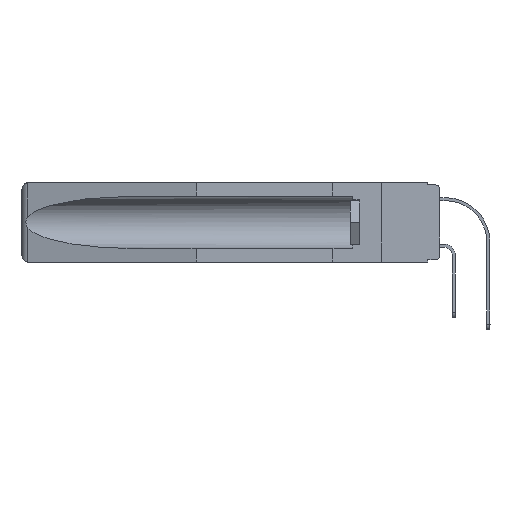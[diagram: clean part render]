
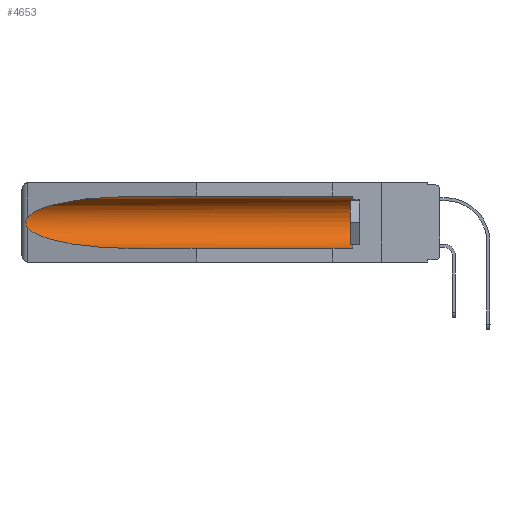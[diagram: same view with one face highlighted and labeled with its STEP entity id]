
A CAD part, left-side view. The second image highlights one B-rep face of the part: STEP entity #4653.
In plain terms, the highlighted cylindrical face has radius 2.857 mm (diameter 5.715 mm), a partial arc.
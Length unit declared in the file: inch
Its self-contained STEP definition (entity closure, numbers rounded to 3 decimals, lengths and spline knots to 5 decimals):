
#161 = ORIENTED_EDGE ( 'NONE', *, *, #1066, .T. ) ;
#438 = CARTESIAN_POINT ( 'NONE',  ( 0.26654, 1.53092, -0.15636 ) ) ;
#1066 = EDGE_CURVE ( 'NONE', #9084, #10188, #7623, .T. ) ;
#1210 = DIRECTION ( 'NONE',  ( 0., -1., 0. ) ) ;
#2127 = VECTOR ( 'NONE', #6569, 39.37008 ) ;
#2269 = ORIENTED_EDGE ( 'NONE', *, *, #20257, .T. ) ;
#2356 = CARTESIAN_POINT ( 'NONE',  ( 0.26537, 1.52718, -0.19328 ) ) ;
#2410 = EDGE_LOOP ( 'NONE', ( #161, #15070, #22019, #6630, #9213, #2269 ) ) ;
#2470 = CARTESIAN_POINT ( 'NONE',  ( 0.2673, 1.53269, -0.17917 ) ) ;
#3411 = VERTEX_POINT ( 'NONE', #25266 ) ;
#3981 = CARTESIAN_POINT ( 'NONE',  ( 0.155, 0.126, -0.059 ) ) ;
#4142 = B_SPLINE_CURVE_WITH_KNOTS ( 'NONE', 3,
 ( #25590, #8987, #438, #17217, #4506, #8713, #2470, #23439, #12776, #16811 ),
 .UNSPECIFIED., .F., .F.,
 ( 4, 2, 2, 2, 4 ),
 ( 0., 0.00029, 0.00058, 0.00087, 0.00117 ),
 .UNSPECIFIED. ) ;
#4506 = CARTESIAN_POINT ( 'NONE',  ( 0.2675, 1.53308, -0.16763 ) ) ;
#4522 = CARTESIAN_POINT ( 'NONE',  ( 0.155, 1.07973, -0.284 ) ) ;
#4653 = ADVANCED_FACE ( 'NONE', ( #8912 ), #9044, .F. ) ;
#5175 = CARTESIAN_POINT ( 'NONE',  ( 0.26537, 1.52718, -0.14972 ) ) ;
#6569 = DIRECTION ( 'NONE',  ( 0., 1., 0. ) ) ;
#6630 = ORIENTED_EDGE ( 'NONE', *, *, #25492, .F. ) ;
#6849 = CARTESIAN_POINT ( 'NONE',  ( 0.155, 1.07973, -0.284 ) ) ;
#6881 = EDGE_CURVE ( 'NONE', #10188, #3411, #4142, .T. ) ;
#7564 = AXIS2_PLACEMENT_3D ( 'NONE', #9723, #1210, #17702 ) ;
#7623 =( BOUNDED_CURVE ( )  B_SPLINE_CURVE ( 3, ( #25746, #15452, #23729, #5175 ),
 .UNSPECIFIED., .F., .F. ) 
 B_SPLINE_CURVE_WITH_KNOTS ( ( 4, 4 ),
 ( 4.71239, 6.08839 ),
 .UNSPECIFIED. ) 
 CURVE ( )  GEOMETRIC_REPRESENTATION_ITEM ( )  RATIONAL_B_SPLINE_CURVE ( ( 1., 0.848, 0.848, 1. ) ) 
 REPRESENTATION_ITEM ( '' )  );
#7659 = EDGE_CURVE ( 'NONE', #3411, #21820, #16913, .T. ) ;
#7836 = AXIS2_PLACEMENT_3D ( 'NONE', #15232, #19451, #21618 ) ;
#7962 = LINE ( 'NONE', #12285, #23637 ) ;
#8355 = EDGE_CURVE ( 'NONE', #23515, #14273, #20101, .T. ) ;
#8713 = CARTESIAN_POINT ( 'NONE',  ( 0.2675, 1.53308, -0.17534 ) ) ;
#8912 = FACE_OUTER_BOUND ( 'NONE', #2410, .T. ) ;
#8987 = CARTESIAN_POINT ( 'NONE',  ( 0.26597, 1.52961, -0.15275 ) ) ;
#9044 = CYLINDRICAL_SURFACE ( 'NONE', #7836, 0.1125 ) ;
#9084 = VERTEX_POINT ( 'NONE', #25361 ) ;
#9213 = ORIENTED_EDGE ( 'NONE', *, *, #8355, .T. ) ;
#9723 = CARTESIAN_POINT ( 'NONE',  ( 0.155, 0.126, -0.1715 ) ) ;
#10188 = VERTEX_POINT ( 'NONE', #21650 ) ;
#12285 = CARTESIAN_POINT ( 'NONE',  ( 0.155, -0.30754, -0.284 ) ) ;
#12520 = CARTESIAN_POINT ( 'NONE',  ( 0.25451, 1.48313, -0.24835 ) ) ;
#12776 = CARTESIAN_POINT ( 'NONE',  ( 0.26597, 1.5296, -0.19026 ) ) ;
#14273 = VERTEX_POINT ( 'NONE', #3981 ) ;
#14536 = CARTESIAN_POINT ( 'NONE',  ( 0.155, 0.126, -0.284 ) ) ;
#15070 = ORIENTED_EDGE ( 'NONE', *, *, #6881, .T. ) ;
#15232 = CARTESIAN_POINT ( 'NONE',  ( 0.155, -0.30754, -0.1715 ) ) ;
#15452 = CARTESIAN_POINT ( 'NONE',  ( 0.21114, 1.30732, -0.059 ) ) ;
#16811 = CARTESIAN_POINT ( 'NONE',  ( 0.26537, 1.52718, -0.19328 ) ) ;
#16913 =( BOUNDED_CURVE ( )  B_SPLINE_CURVE ( 3, ( #2356, #12520, #21305, #4522 ),
 .UNSPECIFIED., .F., .F. ) 
 B_SPLINE_CURVE_WITH_KNOTS ( ( 4, 4 ),
 ( 0.1948, 1.5708 ),
 .UNSPECIFIED. ) 
 CURVE ( )  GEOMETRIC_REPRESENTATION_ITEM ( )  RATIONAL_B_SPLINE_CURVE ( ( 1., 0.848, 0.848, 1. ) ) 
 REPRESENTATION_ITEM ( '' )  );
#17217 = CARTESIAN_POINT ( 'NONE',  ( 0.2673, 1.5327, -0.16383 ) ) ;
#17702 = DIRECTION ( 'NONE',  ( 0., 0., 1. ) ) ;
#18633 = DIRECTION ( 'NONE',  ( 0., 1., 0. ) ) ;
#19451 = DIRECTION ( 'NONE',  ( 0., 1., 0. ) ) ;
#20101 = CIRCLE ( 'NONE', #7564, 0.1125 ) ;
#20257 = EDGE_CURVE ( 'NONE', #14273, #9084, #26714, .T. ) ;
#21305 = CARTESIAN_POINT ( 'NONE',  ( 0.21114, 1.30732, -0.284 ) ) ;
#21618 = DIRECTION ( 'NONE',  ( 0., 0., 1. ) ) ;
#21650 = CARTESIAN_POINT ( 'NONE',  ( 0.26537, 1.52718, -0.14972 ) ) ;
#21820 = VERTEX_POINT ( 'NONE', #6849 ) ;
#22019 = ORIENTED_EDGE ( 'NONE', *, *, #7659, .T. ) ;
#23439 = CARTESIAN_POINT ( 'NONE',  ( 0.26655, 1.53094, -0.18657 ) ) ;
#23515 = VERTEX_POINT ( 'NONE', #14536 ) ;
#23637 = VECTOR ( 'NONE', #18633, 39.37008 ) ;
#23729 = CARTESIAN_POINT ( 'NONE',  ( 0.25451, 1.48313, -0.09465 ) ) ;
#25105 = CARTESIAN_POINT ( 'NONE',  ( 0.155, -0.30754, -0.059 ) ) ;
#25266 = CARTESIAN_POINT ( 'NONE',  ( 0.26537, 1.52718, -0.19328 ) ) ;
#25361 = CARTESIAN_POINT ( 'NONE',  ( 0.155, 1.07973, -0.059 ) ) ;
#25492 = EDGE_CURVE ( 'NONE', #23515, #21820, #7962, .T. ) ;
#25590 = CARTESIAN_POINT ( 'NONE',  ( 0.26537, 1.52718, -0.14972 ) ) ;
#25746 = CARTESIAN_POINT ( 'NONE',  ( 0.155, 1.07973, -0.059 ) ) ;
#26714 = LINE ( 'NONE', #25105, #2127 ) ;
